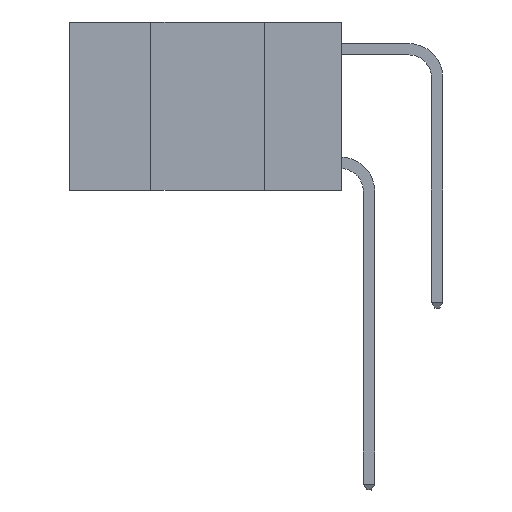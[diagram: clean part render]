
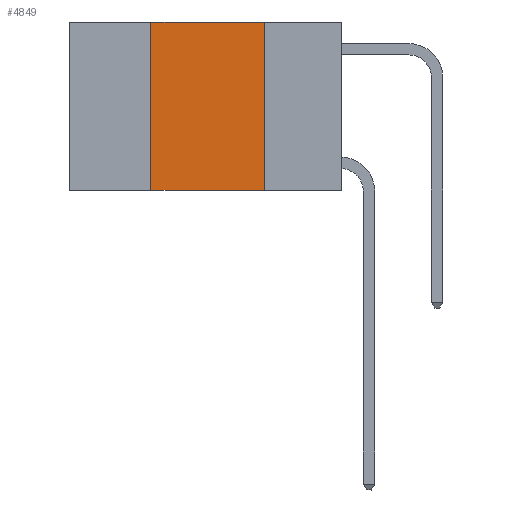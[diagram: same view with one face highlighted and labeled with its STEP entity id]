
A CAD part, left-side view. The second image highlights one B-rep face of the part: STEP entity #4849.
In plain terms, the highlighted planar face has unit normal (-1, 0, 0).
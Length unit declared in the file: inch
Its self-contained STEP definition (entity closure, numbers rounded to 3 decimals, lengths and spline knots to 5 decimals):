
#16 = CARTESIAN_POINT ( 'NONE',  ( 0., 0.17, -0.37 ) ) ;
#464 = VERTEX_POINT ( 'NONE', #3853 ) ;
#1015 = LINE ( 'NONE', #11431, #10419 ) ;
#1906 = ORIENTED_EDGE ( 'NONE', *, *, #7041, .F. ) ;
#2045 = VECTOR ( 'NONE', #4590, 39.37008 ) ;
#2185 = ORIENTED_EDGE ( 'NONE', *, *, #9510, .T. ) ;
#2561 = VERTEX_POINT ( 'NONE', #5702 ) ;
#2783 = DIRECTION ( 'NONE',  ( 0., -1., 0. ) ) ;
#2928 = LINE ( 'NONE', #10889, #7564 ) ;
#3853 = CARTESIAN_POINT ( 'NONE',  ( 0., 0.42, -0.37 ) ) ;
#4590 = DIRECTION ( 'NONE',  ( 0., -1., 0. ) ) ;
#4821 = VECTOR ( 'NONE', #2783, 39.37008 ) ;
#4849 = ADVANCED_FACE ( 'NONE', ( #5811 ), #5408, .F. ) ;
#4976 = VERTEX_POINT ( 'NONE', #9511 ) ;
#5128 = LINE ( 'NONE', #10049, #4821 ) ;
#5408 = PLANE ( 'NONE',  #8872 ) ;
#5702 = CARTESIAN_POINT ( 'NONE',  ( 0., 0.42, 0. ) ) ;
#5811 = FACE_OUTER_BOUND ( 'NONE', #7956, .T. ) ;
#6181 = CARTESIAN_POINT ( 'NONE',  ( 0., 0.6, 0. ) ) ;
#6295 = DIRECTION ( 'NONE',  ( 0., 0., -1. ) ) ;
#6848 = EDGE_CURVE ( 'NONE', #4976, #9562, #1015, .T. ) ;
#7041 = EDGE_CURVE ( 'NONE', #2561, #4976, #9068, .T. ) ;
#7369 = DIRECTION ( 'NONE',  ( 0., 0., 1. ) ) ;
#7564 = VECTOR ( 'NONE', #7369, 39.37008 ) ;
#7956 = EDGE_LOOP ( 'NONE', ( #11186, #1906, #9206, #2185 ) ) ;
#8872 = AXIS2_PLACEMENT_3D ( 'NONE', #6181, #11489, #6295 ) ;
#9068 = LINE ( 'NONE', #11655, #2045 ) ;
#9206 = ORIENTED_EDGE ( 'NONE', *, *, #10886, .F. ) ;
#9510 = EDGE_CURVE ( 'NONE', #464, #9562, #5128, .T. ) ;
#9511 = CARTESIAN_POINT ( 'NONE',  ( 0., 0.17, 0. ) ) ;
#9562 = VERTEX_POINT ( 'NONE', #16 ) ;
#9783 = DIRECTION ( 'NONE',  ( 0., 0., -1. ) ) ;
#10049 = CARTESIAN_POINT ( 'NONE',  ( 0., 0.6, -0.37 ) ) ;
#10419 = VECTOR ( 'NONE', #9783, 39.37008 ) ;
#10886 = EDGE_CURVE ( 'NONE', #464, #2561, #2928, .T. ) ;
#10889 = CARTESIAN_POINT ( 'NONE',  ( 0., 0.42, 0. ) ) ;
#11186 = ORIENTED_EDGE ( 'NONE', *, *, #6848, .F. ) ;
#11431 = CARTESIAN_POINT ( 'NONE',  ( 0., 0.17, 0. ) ) ;
#11489 = DIRECTION ( 'NONE',  ( 1., 0., 0. ) ) ;
#11655 = CARTESIAN_POINT ( 'NONE',  ( 0., 0.6, 0. ) ) ;
